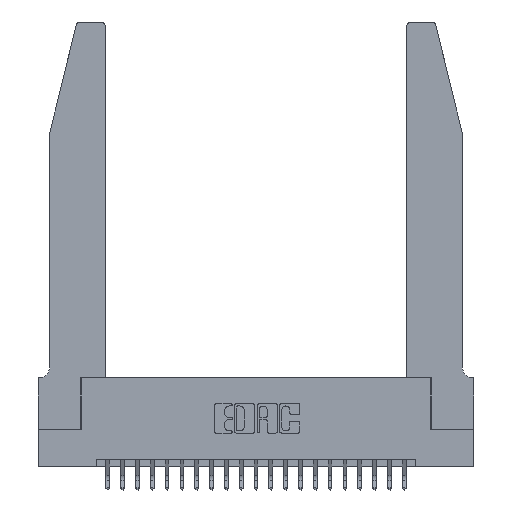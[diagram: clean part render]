
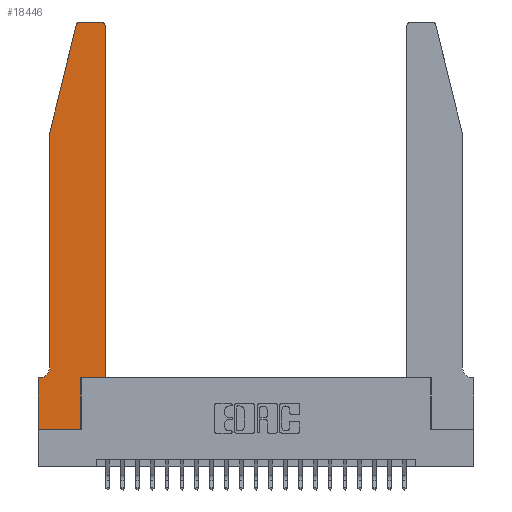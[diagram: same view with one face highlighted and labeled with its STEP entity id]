
A CAD part, top view. The second image highlights one B-rep face of the part: STEP entity #18446.
In plain terms, the highlighted planar face has unit normal (0, 0, 1).
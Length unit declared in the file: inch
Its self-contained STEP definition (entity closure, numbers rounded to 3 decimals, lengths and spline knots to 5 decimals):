
#171 = DIRECTION ( 'NONE',  ( -1., 0., 0. ) ) ;
#474 = VECTOR ( 'NONE', #22381, 39.37008 ) ;
#566 = EDGE_CURVE ( 'NONE', #4283, #21275, #15892, .T. ) ;
#1332 = VERTEX_POINT ( 'NONE', #11685 ) ;
#1372 = CARTESIAN_POINT ( 'NONE',  ( 0.0755, 0.35, 0.37 ) ) ;
#1518 = CARTESIAN_POINT ( 'NONE',  ( 0.0755, 2., 0.37 ) ) ;
#1581 = ORIENTED_EDGE ( 'NONE', *, *, #13357, .T. ) ;
#1683 = CARTESIAN_POINT ( 'NONE',  ( 0.0755, 2., 0.37 ) ) ;
#1691 = VERTEX_POINT ( 'NONE', #5755 ) ;
#1769 = CIRCLE ( 'NONE', #4321, 0.07 ) ;
#1785 = DIRECTION ( 'NONE',  ( 0., 0., 1. ) ) ;
#1863 = DIRECTION ( 'NONE',  ( 1., 0., 0. ) ) ;
#1986 = CARTESIAN_POINT ( 'NONE',  ( 0.4205, 2.72, 0.37 ) ) ;
#2393 = CARTESIAN_POINT ( 'NONE',  ( 0., 0., 0.37 ) ) ;
#2701 = CARTESIAN_POINT ( 'NONE',  ( 0.0055, 0.35, 0.37 ) ) ;
#3563 = AXIS2_PLACEMENT_3D ( 'NONE', #16151, #10560, #5062 ) ;
#3691 = ORIENTED_EDGE ( 'NONE', *, *, #15520, .T. ) ;
#3860 = VECTOR ( 'NONE', #20415, 39.37008 ) ;
#3881 = EDGE_CURVE ( 'NONE', #8686, #1332, #15895, .T. ) ;
#4283 = VERTEX_POINT ( 'NONE', #18758 ) ;
#4321 = AXIS2_PLACEMENT_3D ( 'NONE', #11429, #5843, #171 ) ;
#4718 = EDGE_CURVE ( 'NONE', #9708, #18210, #17941, .T. ) ;
#4772 = EDGE_CURVE ( 'NONE', #24000, #13323, #22586, .T. ) ;
#4874 = EDGE_CURVE ( 'NONE', #21275, #7608, #6440, .T. ) ;
#5062 = DIRECTION ( 'NONE',  ( 1., 0., 0. ) ) ;
#5755 = CARTESIAN_POINT ( 'NONE',  ( 0.4505, 2.72, 0.37 ) ) ;
#5843 = DIRECTION ( 'NONE',  ( 0., 0., -1. ) ) ;
#5954 = DIRECTION ( 'NONE',  ( -1., 0., 0. ) ) ;
#6164 = VECTOR ( 'NONE', #14517, 39.37008 ) ;
#6440 = LINE ( 'NONE', #14761, #23759 ) ;
#7052 = CARTESIAN_POINT ( 'NONE',  ( 0.4205, 2.75, 0.37 ) ) ;
#7384 = CARTESIAN_POINT ( 'NONE',  ( 0.4505, 0.35, 0.37 ) ) ;
#7432 = CARTESIAN_POINT ( 'NONE',  ( 0.2605, 2.75, 0.37 ) ) ;
#7608 = VERTEX_POINT ( 'NONE', #19765 ) ;
#7907 = EDGE_CURVE ( 'NONE', #1332, #4283, #17195, .T. ) ;
#8549 = VECTOR ( 'NONE', #11132, 39.37008 ) ;
#8686 = VERTEX_POINT ( 'NONE', #20939 ) ;
#8873 = ORIENTED_EDGE ( 'NONE', *, *, #15044, .T. ) ;
#9250 = LINE ( 'NONE', #7384, #474 ) ;
#9520 = VERTEX_POINT ( 'NONE', #2701 ) ;
#9668 = CARTESIAN_POINT ( 'NONE',  ( 0.0755, 0.42, 0.37 ) ) ;
#9708 = VERTEX_POINT ( 'NONE', #12879 ) ;
#10036 = CARTESIAN_POINT ( 'NONE',  ( 0.2865, 0.35, 0.37 ) ) ;
#10560 = DIRECTION ( 'NONE',  ( 0., 0., 1. ) ) ;
#10909 = DIRECTION ( 'NONE',  ( -1., 0., 0. ) ) ;
#11132 = DIRECTION ( 'NONE',  ( -0.239, -0.971, 0. ) ) ;
#11429 = CARTESIAN_POINT ( 'NONE',  ( 0.0055, 0.42, 0.37 ) ) ;
#11591 = VECTOR ( 'NONE', #20491, 39.37008 ) ;
#11685 = CARTESIAN_POINT ( 'NONE',  ( 0., 0., 0.37 ) ) ;
#12079 = ORIENTED_EDGE ( 'NONE', *, *, #7907, .T. ) ;
#12237 = CARTESIAN_POINT ( 'NONE',  ( 0.25487, 2.72718, 0.37 ) ) ;
#12523 = EDGE_CURVE ( 'NONE', #9520, #8686, #12706, .T. ) ;
#12706 = LINE ( 'NONE', #1372, #23530 ) ;
#12815 = LINE ( 'NONE', #7432, #19530 ) ;
#12879 = CARTESIAN_POINT ( 'NONE',  ( 0.284, 2.75, 0.37 ) ) ;
#13121 = CARTESIAN_POINT ( 'NONE',  ( 0., 0.35, 0.37 ) ) ;
#13149 = ORIENTED_EDGE ( 'NONE', *, *, #4874, .T. ) ;
#13150 = CIRCLE ( 'NONE', #19415, 0.03 ) ;
#13258 = DIRECTION ( 'NONE',  ( 1., 0., 0. ) ) ;
#13323 = VERTEX_POINT ( 'NONE', #9668 ) ;
#13357 = EDGE_CURVE ( 'NONE', #13323, #9520, #1769, .T. ) ;
#13899 = FACE_OUTER_BOUND ( 'NONE', #22089, .T. ) ;
#13968 = ORIENTED_EDGE ( 'NONE', *, *, #4718, .T. ) ;
#14517 = DIRECTION ( 'NONE',  ( 0., -1., 0. ) ) ;
#14602 = CARTESIAN_POINT ( 'NONE',  ( 0.0755, 2., 0.37 ) ) ;
#14754 = LINE ( 'NONE', #1518, #8549 ) ;
#14761 = CARTESIAN_POINT ( 'NONE',  ( 0.4505, 0.35, 0.37 ) ) ;
#15044 = EDGE_CURVE ( 'NONE', #1691, #15372, #13150, .T. ) ;
#15067 = ORIENTED_EDGE ( 'NONE', *, *, #566, .T. ) ;
#15372 = VERTEX_POINT ( 'NONE', #7052 ) ;
#15520 = EDGE_CURVE ( 'NONE', #7608, #1691, #9250, .T. ) ;
#15534 = DIRECTION ( 'NONE',  ( 0., -1., 0. ) ) ;
#15892 = LINE ( 'NONE', #18547, #3860 ) ;
#15895 = LINE ( 'NONE', #2393, #23495 ) ;
#16151 = CARTESIAN_POINT ( 'NONE',  ( 0.284, 2.72, 0.37 ) ) ;
#16656 = DIRECTION ( 'NONE',  ( 1., 0., 0. ) ) ;
#17195 = LINE ( 'NONE', #20652, #11591 ) ;
#17552 = ORIENTED_EDGE ( 'NONE', *, *, #12523, .T. ) ;
#17600 = ORIENTED_EDGE ( 'NONE', *, *, #3881, .T. ) ;
#17941 = CIRCLE ( 'NONE', #3563, 0.03 ) ;
#18210 = VERTEX_POINT ( 'NONE', #12237 ) ;
#18446 = ADVANCED_FACE ( 'NONE', ( #13899 ), #19848, .T. ) ;
#18547 = CARTESIAN_POINT ( 'NONE',  ( 0.2865, 0.35, 0.37 ) ) ;
#18693 = ORIENTED_EDGE ( 'NONE', *, *, #19047, .T. ) ;
#18721 = ORIENTED_EDGE ( 'NONE', *, *, #22231, .T. ) ;
#18758 = CARTESIAN_POINT ( 'NONE',  ( 0.2865, 0., 0.37 ) ) ;
#19047 = EDGE_CURVE ( 'NONE', #18210, #24000, #14754, .T. ) ;
#19415 = AXIS2_PLACEMENT_3D ( 'NONE', #1986, #22733, #13258 ) ;
#19530 = VECTOR ( 'NONE', #5954, 39.37008 ) ;
#19765 = CARTESIAN_POINT ( 'NONE',  ( 0.4505, 0.35, 0.37 ) ) ;
#19848 = PLANE ( 'NONE',  #23847 ) ;
#20415 = DIRECTION ( 'NONE',  ( 0., 1., 0. ) ) ;
#20491 = DIRECTION ( 'NONE',  ( 1., 0., 0. ) ) ;
#20652 = CARTESIAN_POINT ( 'NONE',  ( 0., 0., 0.37 ) ) ;
#20939 = CARTESIAN_POINT ( 'NONE',  ( 0., 0.35, 0.37 ) ) ;
#21189 = ORIENTED_EDGE ( 'NONE', *, *, #4772, .T. ) ;
#21275 = VERTEX_POINT ( 'NONE', #10036 ) ;
#22089 = EDGE_LOOP ( 'NONE', ( #18721, #13968, #18693, #21189, #1581, #17552, #17600, #12079, #15067, #13149, #3691, #8873 ) ) ;
#22231 = EDGE_CURVE ( 'NONE', #15372, #9708, #12815, .T. ) ;
#22381 = DIRECTION ( 'NONE',  ( 0., 1., 0. ) ) ;
#22586 = LINE ( 'NONE', #14602, #6164 ) ;
#22733 = DIRECTION ( 'NONE',  ( 0., 0., 1. ) ) ;
#23495 = VECTOR ( 'NONE', #15534, 39.37008 ) ;
#23530 = VECTOR ( 'NONE', #10909, 39.37008 ) ;
#23759 = VECTOR ( 'NONE', #16656, 39.37008 ) ;
#23847 = AXIS2_PLACEMENT_3D ( 'NONE', #13121, #1785, #1863 ) ;
#24000 = VERTEX_POINT ( 'NONE', #1683 ) ;
